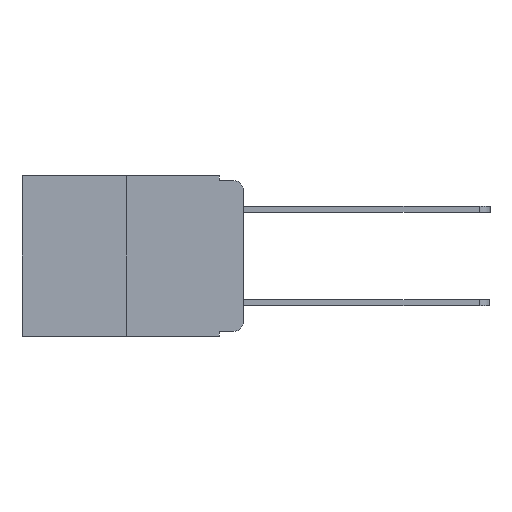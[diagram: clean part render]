
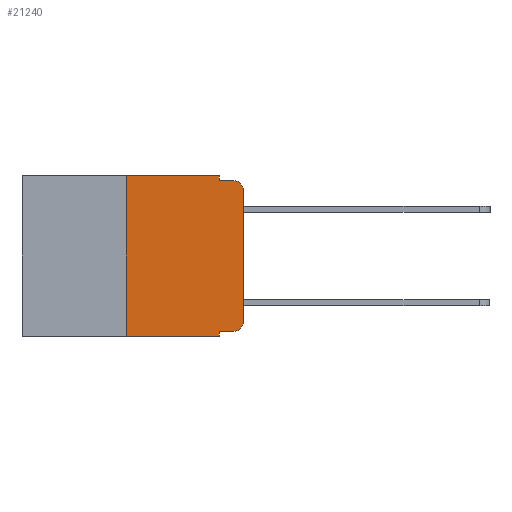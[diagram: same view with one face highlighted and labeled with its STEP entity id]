
A CAD part, left-side view. The second image highlights one B-rep face of the part: STEP entity #21240.
In plain terms, the highlighted planar face has unit normal (-1, 0, 0).
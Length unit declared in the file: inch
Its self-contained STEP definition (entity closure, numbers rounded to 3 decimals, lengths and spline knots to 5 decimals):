
#216 = VERTEX_POINT ( 'NONE', #12235 ) ;
#656 = VECTOR ( 'NONE', #7685, 39.37008 ) ;
#986 = DIRECTION ( 'NONE',  ( 0., 0., -1. ) ) ;
#1195 = LINE ( 'NONE', #6020, #656 ) ;
#1211 = FACE_OUTER_BOUND ( 'NONE', #5227, .T. ) ;
#1253 = DIRECTION ( 'NONE',  ( -1., 0., 0. ) ) ;
#1335 = EDGE_CURVE ( 'NONE', #216, #19991, #6479, .T. ) ;
#1493 = EDGE_CURVE ( 'NONE', #13130, #11888, #3306, .T. ) ;
#1517 = ORIENTED_EDGE ( 'NONE', *, *, #2032, .F. ) ;
#1872 = LINE ( 'NONE', #8085, #10362 ) ;
#1882 = DIRECTION ( 'NONE',  ( 1., 0., 0. ) ) ;
#2032 = EDGE_CURVE ( 'NONE', #5045, #6968, #4702, .T. ) ;
#2262 = CARTESIAN_POINT ( 'NONE',  ( 0., 0., 0. ) ) ;
#2483 = VECTOR ( 'NONE', #17814, 39.37008 ) ;
#2843 = ORIENTED_EDGE ( 'NONE', *, *, #7285, .F. ) ;
#2863 = ORIENTED_EDGE ( 'NONE', *, *, #4416, .T. ) ;
#3306 = CIRCLE ( 'NONE', #4008, 0.02 ) ;
#3414 = ORIENTED_EDGE ( 'NONE', *, *, #19021, .F. ) ;
#4008 = AXIS2_PLACEMENT_3D ( 'NONE', #13911, #13879, #13859 ) ;
#4416 = EDGE_CURVE ( 'NONE', #216, #21180, #12825, .T. ) ;
#4702 = LINE ( 'NONE', #15984, #13653 ) ;
#4977 = CARTESIAN_POINT ( 'NONE',  ( 0., 0., -0.03 ) ) ;
#5045 = VERTEX_POINT ( 'NONE', #14617 ) ;
#5227 = EDGE_LOOP ( 'NONE', ( #13645, #14167, #2843, #1517, #11072, #5258, #2863, #3414, #10017, #10564 ) ) ;
#5258 = ORIENTED_EDGE ( 'NONE', *, *, #1335, .F. ) ;
#5445 = CIRCLE ( 'NONE', #6276, 0.02 ) ;
#5594 = CARTESIAN_POINT ( 'NONE',  ( 0., 0.051, -0.01 ) ) ;
#5852 = VERTEX_POINT ( 'NONE', #19899 ) ;
#6020 = CARTESIAN_POINT ( 'NONE',  ( 0., 0.051, 0. ) ) ;
#6094 = VECTOR ( 'NONE', #6468, 39.37008 ) ;
#6276 = AXIS2_PLACEMENT_3D ( 'NONE', #11378, #1253, #13086 ) ;
#6279 = CARTESIAN_POINT ( 'NONE',  ( 0., 0.473, -0.343 ) ) ;
#6331 = EDGE_CURVE ( 'NONE', #8225, #13130, #11680, .T. ) ;
#6468 = DIRECTION ( 'NONE',  ( 0., -1., 0. ) ) ;
#6479 = LINE ( 'NONE', #17052, #2483 ) ;
#6639 = EDGE_CURVE ( 'NONE', #19991, #5045, #1872, .T. ) ;
#6717 = EDGE_CURVE ( 'NONE', #12138, #5852, #8758, .T. ) ;
#6968 = VERTEX_POINT ( 'NONE', #5594 ) ;
#7222 = CARTESIAN_POINT ( 'NONE',  ( 0., 0.25, 0. ) ) ;
#7285 = EDGE_CURVE ( 'NONE', #6968, #11888, #10601, .T. ) ;
#7685 = DIRECTION ( 'NONE',  ( 0., 0., -1. ) ) ;
#7950 = DIRECTION ( 'NONE',  ( 0., -1., 0. ) ) ;
#8085 = CARTESIAN_POINT ( 'NONE',  ( 0., 0.473, 0. ) ) ;
#8225 = VERTEX_POINT ( 'NONE', #18841 ) ;
#8320 = VECTOR ( 'NONE', #7950, 39.37008 ) ;
#8758 = LINE ( 'NONE', #19945, #21427 ) ;
#9818 = DIRECTION ( 'NONE',  ( 0., -1., 0. ) ) ;
#10017 = ORIENTED_EDGE ( 'NONE', *, *, #6717, .T. ) ;
#10362 = VECTOR ( 'NONE', #9818, 39.37008 ) ;
#10564 = ORIENTED_EDGE ( 'NONE', *, *, #11655, .T. ) ;
#10601 = LINE ( 'NONE', #13176, #6094 ) ;
#10725 = DIRECTION ( 'NONE',  ( 0., 0., 1. ) ) ;
#11072 = ORIENTED_EDGE ( 'NONE', *, *, #6639, .F. ) ;
#11378 = CARTESIAN_POINT ( 'NONE',  ( 0., 0.02, -0.313 ) ) ;
#11655 = EDGE_CURVE ( 'NONE', #5852, #8225, #5445, .T. ) ;
#11680 = LINE ( 'NONE', #2262, #16097 ) ;
#11798 = CARTESIAN_POINT ( 'NONE',  ( 0., 0.051, -0.343 ) ) ;
#11888 = VERTEX_POINT ( 'NONE', #20174 ) ;
#12020 = CARTESIAN_POINT ( 'NONE',  ( 0., 0.473, 0. ) ) ;
#12138 = VERTEX_POINT ( 'NONE', #15867 ) ;
#12235 = CARTESIAN_POINT ( 'NONE',  ( 0., 0.25, -0.343 ) ) ;
#12825 = LINE ( 'NONE', #6279, #8320 ) ;
#13086 = DIRECTION ( 'NONE',  ( 0., 0., -1. ) ) ;
#13130 = VERTEX_POINT ( 'NONE', #4977 ) ;
#13176 = CARTESIAN_POINT ( 'NONE',  ( 0., 0.051, -0.01 ) ) ;
#13645 = ORIENTED_EDGE ( 'NONE', *, *, #6331, .T. ) ;
#13653 = VECTOR ( 'NONE', #986, 39.37008 ) ;
#13679 = DIRECTION ( 'NONE',  ( 0., 0., -1. ) ) ;
#13859 = DIRECTION ( 'NONE',  ( 0., 0., -1. ) ) ;
#13879 = DIRECTION ( 'NONE',  ( -1., 0., 0. ) ) ;
#13911 = CARTESIAN_POINT ( 'NONE',  ( 0., 0.02, -0.03 ) ) ;
#14167 = ORIENTED_EDGE ( 'NONE', *, *, #1493, .T. ) ;
#14617 = CARTESIAN_POINT ( 'NONE',  ( 0., 0.051, 0. ) ) ;
#15867 = CARTESIAN_POINT ( 'NONE',  ( 0., 0.051, -0.333 ) ) ;
#15984 = CARTESIAN_POINT ( 'NONE',  ( 0., 0.051, 0. ) ) ;
#16097 = VECTOR ( 'NONE', #10725, 39.37008 ) ;
#17052 = CARTESIAN_POINT ( 'NONE',  ( 0., 0.25, 0. ) ) ;
#17814 = DIRECTION ( 'NONE',  ( 0., 0., 1. ) ) ;
#18313 = DIRECTION ( 'NONE',  ( 0., -1., 0. ) ) ;
#18582 = AXIS2_PLACEMENT_3D ( 'NONE', #12020, #1882, #13679 ) ;
#18841 = CARTESIAN_POINT ( 'NONE',  ( 0., 0., -0.313 ) ) ;
#19021 = EDGE_CURVE ( 'NONE', #12138, #21180, #1195, .T. ) ;
#19899 = CARTESIAN_POINT ( 'NONE',  ( 0., 0.02, -0.333 ) ) ;
#19945 = CARTESIAN_POINT ( 'NONE',  ( 0., 0.051, -0.333 ) ) ;
#19991 = VERTEX_POINT ( 'NONE', #7222 ) ;
#20174 = CARTESIAN_POINT ( 'NONE',  ( 0., 0.02, -0.01 ) ) ;
#20239 = PLANE ( 'NONE',  #18582 ) ;
#21180 = VERTEX_POINT ( 'NONE', #11798 ) ;
#21240 = ADVANCED_FACE ( 'NONE', ( #1211 ), #20239, .F. ) ;
#21427 = VECTOR ( 'NONE', #18313, 39.37008 ) ;
